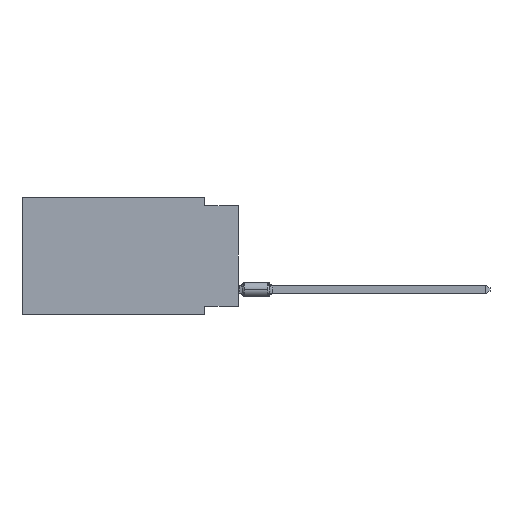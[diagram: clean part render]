
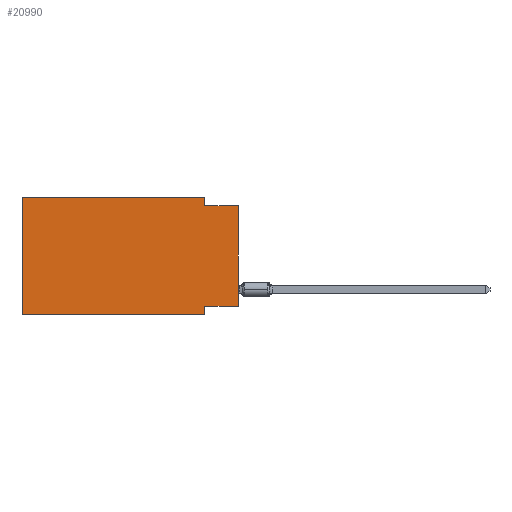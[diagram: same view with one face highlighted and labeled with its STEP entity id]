
A CAD part, left-side view. The second image highlights one B-rep face of the part: STEP entity #20990.
In plain terms, the highlighted planar face has unit normal (-1, 0, 0).
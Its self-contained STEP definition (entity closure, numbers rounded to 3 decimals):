
#11 = EDGE_CURVE ( 'NONE', #15855, #2154, #8846, .T. ) ;
#531 = VERTEX_POINT ( 'NONE', #4457 ) ;
#664 = EDGE_CURVE ( 'NONE', #531, #13828, #5293, .T. ) ;
#786 = CARTESIAN_POINT ( 'NONE',  ( 0., 16.383, -8.89 ) ) ;
#1314 = CARTESIAN_POINT ( 'NONE',  ( 0., 0., 0. ) ) ;
#1400 = ORIENTED_EDGE ( 'NONE', *, *, #8158, .F. ) ;
#2095 = VERTEX_POINT ( 'NONE', #23852 ) ;
#2154 = VERTEX_POINT ( 'NONE', #5912 ) ;
#2347 = CARTESIAN_POINT ( 'NONE',  ( 0., 16.383, 0. ) ) ;
#2728 = EDGE_LOOP ( 'NONE', ( #3298, #17204, #4344, #5098, #1400, #10480, #4591, #14545 ) ) ;
#3105 = LINE ( 'NONE', #8656, #21807 ) ;
#3298 = ORIENTED_EDGE ( 'NONE', *, *, #14304, .T. ) ;
#3592 = DIRECTION ( 'NONE',  ( 0., 0., -1. ) ) ;
#4255 = CARTESIAN_POINT ( 'NONE',  ( 0., 0., -0.635 ) ) ;
#4344 = ORIENTED_EDGE ( 'NONE', *, *, #23311, .F. ) ;
#4457 = CARTESIAN_POINT ( 'NONE',  ( 0., 0., -8.255 ) ) ;
#4469 = CARTESIAN_POINT ( 'NONE',  ( 0., 16.383, 0. ) ) ;
#4591 = ORIENTED_EDGE ( 'NONE', *, *, #23076, .F. ) ;
#5098 = ORIENTED_EDGE ( 'NONE', *, *, #11, .F. ) ;
#5293 = LINE ( 'NONE', #23348, #13104 ) ;
#5433 = CARTESIAN_POINT ( 'NONE',  ( 0., 2.54, -8.89 ) ) ;
#5821 = CARTESIAN_POINT ( 'NONE',  ( 0., 0., -0.635 ) ) ;
#5912 = CARTESIAN_POINT ( 'NONE',  ( 0., 2.54, 0. ) ) ;
#6079 = LINE ( 'NONE', #4255, #10040 ) ;
#6153 = LINE ( 'NONE', #19101, #6868 ) ;
#6491 = CARTESIAN_POINT ( 'NONE',  ( 0., 16.383, 0. ) ) ;
#6868 = VECTOR ( 'NONE', #15354, 1000. ) ;
#7620 = EDGE_CURVE ( 'NONE', #2095, #11474, #6079, .T. ) ;
#8132 = DIRECTION ( 'NONE',  ( 0., -1., 0. ) ) ;
#8158 = EDGE_CURVE ( 'NONE', #17331, #15855, #21056, .T. ) ;
#8231 = CARTESIAN_POINT ( 'NONE',  ( 0., 2.54, -8.89 ) ) ;
#8637 = VECTOR ( 'NONE', #11960, 1000. ) ;
#8656 = CARTESIAN_POINT ( 'NONE',  ( 0., 16.383, -8.89 ) ) ;
#8846 = LINE ( 'NONE', #16229, #20917 ) ;
#9188 = LINE ( 'NONE', #5433, #10716 ) ;
#9611 = CARTESIAN_POINT ( 'NONE',  ( 0., 2.54, -8.255 ) ) ;
#10040 = VECTOR ( 'NONE', #8132, 1000. ) ;
#10480 = ORIENTED_EDGE ( 'NONE', *, *, #14753, .T. ) ;
#10716 = VECTOR ( 'NONE', #20329, 1000. ) ;
#10848 = DIRECTION ( 'NONE',  ( 1., 0., 0. ) ) ;
#11474 = VERTEX_POINT ( 'NONE', #5821 ) ;
#11960 = DIRECTION ( 'NONE',  ( 0., 0., 1. ) ) ;
#13104 = VECTOR ( 'NONE', #21766, 1000. ) ;
#13828 = VERTEX_POINT ( 'NONE', #9611 ) ;
#14304 = EDGE_CURVE ( 'NONE', #531, #11474, #21533, .T. ) ;
#14545 = ORIENTED_EDGE ( 'NONE', *, *, #664, .F. ) ;
#14726 = FACE_OUTER_BOUND ( 'NONE', #2728, .T. ) ;
#14753 = EDGE_CURVE ( 'NONE', #17331, #17543, #3105, .T. ) ;
#15354 = DIRECTION ( 'NONE',  ( 0., 0., -1. ) ) ;
#15731 = VECTOR ( 'NONE', #22513, 1000. ) ;
#15855 = VERTEX_POINT ( 'NONE', #6491 ) ;
#16229 = CARTESIAN_POINT ( 'NONE',  ( 0., 16.383, 0. ) ) ;
#16436 = AXIS2_PLACEMENT_3D ( 'NONE', #2347, #10848, #3592 ) ;
#17204 = ORIENTED_EDGE ( 'NONE', *, *, #7620, .F. ) ;
#17331 = VERTEX_POINT ( 'NONE', #786 ) ;
#17543 = VERTEX_POINT ( 'NONE', #8231 ) ;
#18806 = PLANE ( 'NONE',  #16436 ) ;
#19101 = CARTESIAN_POINT ( 'NONE',  ( 0., 2.54, 0. ) ) ;
#20329 = DIRECTION ( 'NONE',  ( 0., 0., -1. ) ) ;
#20917 = VECTOR ( 'NONE', #23614, 1000. ) ;
#20990 = ADVANCED_FACE ( 'NONE', ( #14726 ), #18806, .F. ) ;
#21056 = LINE ( 'NONE', #4469, #15731 ) ;
#21372 = DIRECTION ( 'NONE',  ( 0., -1., 0. ) ) ;
#21533 = LINE ( 'NONE', #1314, #8637 ) ;
#21766 = DIRECTION ( 'NONE',  ( 0., 1., 0. ) ) ;
#21807 = VECTOR ( 'NONE', #21372, 1000. ) ;
#22513 = DIRECTION ( 'NONE',  ( 0., 0., 1. ) ) ;
#23076 = EDGE_CURVE ( 'NONE', #13828, #17543, #9188, .T. ) ;
#23311 = EDGE_CURVE ( 'NONE', #2154, #2095, #6153, .T. ) ;
#23348 = CARTESIAN_POINT ( 'NONE',  ( 0., 0., -8.255 ) ) ;
#23614 = DIRECTION ( 'NONE',  ( 0., -1., 0. ) ) ;
#23852 = CARTESIAN_POINT ( 'NONE',  ( 0., 2.54, -0.635 ) ) ;
